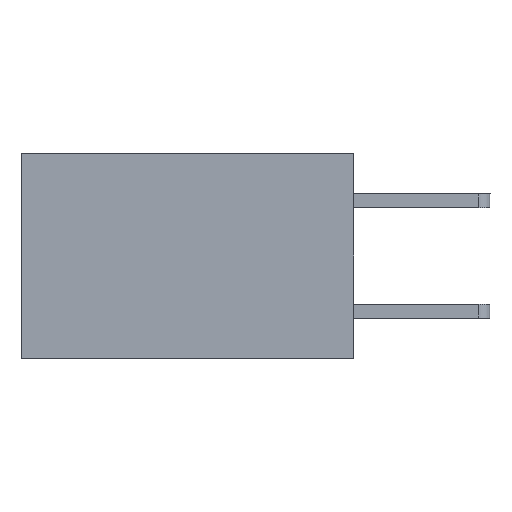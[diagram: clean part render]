
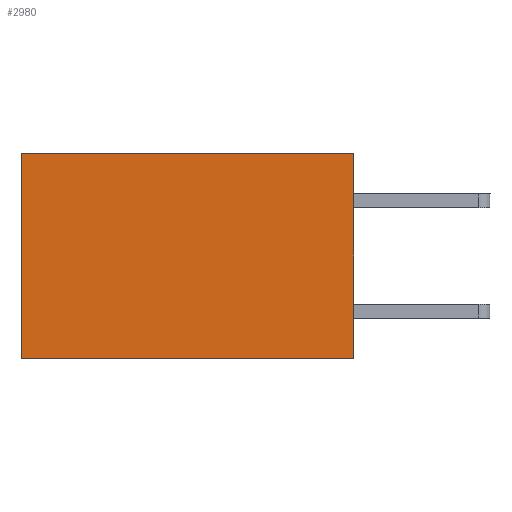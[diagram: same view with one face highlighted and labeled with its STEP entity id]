
A CAD part, left-side view. The second image highlights one B-rep face of the part: STEP entity #2980.
In plain terms, the highlighted planar face has unit normal (-1, 0, 0).
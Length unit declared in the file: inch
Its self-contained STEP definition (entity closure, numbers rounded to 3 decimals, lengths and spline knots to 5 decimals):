
#678 = VERTEX_POINT ( 'NONE', #8245 ) ;
#811 = DIRECTION ( 'NONE',  ( 0., 0., -1. ) ) ;
#984 = ORIENTED_EDGE ( 'NONE', *, *, #2958, .F. ) ;
#1247 = CARTESIAN_POINT ( 'NONE',  ( 0.2875, 0., 0. ) ) ;
#1565 = VECTOR ( 'NONE', #5511, 39.37008 ) ;
#1780 = LINE ( 'NONE', #1247, #3404 ) ;
#2361 = EDGE_CURVE ( 'NONE', #7532, #678, #5850, .T. ) ;
#2772 = ORIENTED_EDGE ( 'NONE', *, *, #2361, .F. ) ;
#2958 = EDGE_CURVE ( 'NONE', #678, #6219, #5104, .T. ) ;
#2980 = ADVANCED_FACE ( 'NONE', ( #9178 ), #9720, .F. ) ;
#3214 = CARTESIAN_POINT ( 'NONE',  ( 0.2875, 0., 0. ) ) ;
#3404 = VECTOR ( 'NONE', #5292, 39.37008 ) ;
#3814 = AXIS2_PLACEMENT_3D ( 'NONE', #8179, #9752, #9836 ) ;
#4124 = CARTESIAN_POINT ( 'NONE',  ( 0.2875, 0., 0. ) ) ;
#4332 = EDGE_CURVE ( 'NONE', #7532, #8083, #1780, .T. ) ;
#4416 = VECTOR ( 'NONE', #811, 39.37008 ) ;
#4714 = DIRECTION ( 'NONE',  ( 0., 1., 0. ) ) ;
#4908 = EDGE_CURVE ( 'NONE', #8083, #6219, #5928, .T. ) ;
#5104 = LINE ( 'NONE', #10395, #5703 ) ;
#5292 = DIRECTION ( 'NONE',  ( 0., 1., 0. ) ) ;
#5511 = DIRECTION ( 'NONE',  ( 0., 0., -1. ) ) ;
#5703 = VECTOR ( 'NONE', #4714, 39.37008 ) ;
#5850 = LINE ( 'NONE', #3214, #1565 ) ;
#5928 = LINE ( 'NONE', #9681, #4416 ) ;
#6179 = ORIENTED_EDGE ( 'NONE', *, *, #4332, .T. ) ;
#6219 = VERTEX_POINT ( 'NONE', #6496 ) ;
#6496 = CARTESIAN_POINT ( 'NONE',  ( 0.2875, 0.6, -0.37 ) ) ;
#7532 = VERTEX_POINT ( 'NONE', #4124 ) ;
#8083 = VERTEX_POINT ( 'NONE', #8524 ) ;
#8179 = CARTESIAN_POINT ( 'NONE',  ( 0.2875, 0., 0. ) ) ;
#8245 = CARTESIAN_POINT ( 'NONE',  ( 0.2875, 0., -0.37 ) ) ;
#8524 = CARTESIAN_POINT ( 'NONE',  ( 0.2875, 0.6, 0. ) ) ;
#8599 = ORIENTED_EDGE ( 'NONE', *, *, #4908, .T. ) ;
#8904 = EDGE_LOOP ( 'NONE', ( #8599, #984, #2772, #6179 ) ) ;
#9178 = FACE_OUTER_BOUND ( 'NONE', #8904, .T. ) ;
#9681 = CARTESIAN_POINT ( 'NONE',  ( 0.2875, 0.6, 0. ) ) ;
#9720 = PLANE ( 'NONE',  #3814 ) ;
#9752 = DIRECTION ( 'NONE',  ( 1., 0., 0. ) ) ;
#9836 = DIRECTION ( 'NONE',  ( 0., 0., -1. ) ) ;
#10395 = CARTESIAN_POINT ( 'NONE',  ( 0.2875, 0., -0.37 ) ) ;
